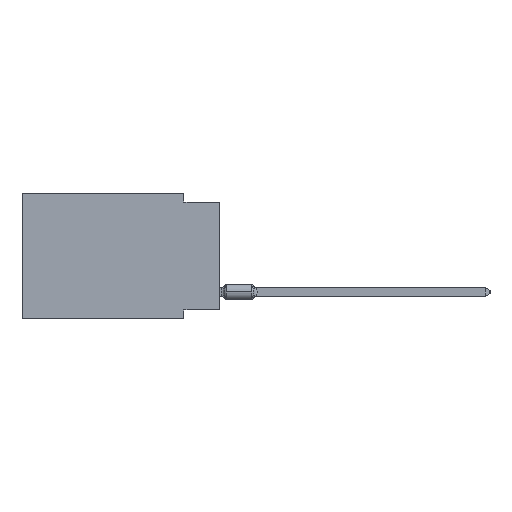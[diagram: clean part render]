
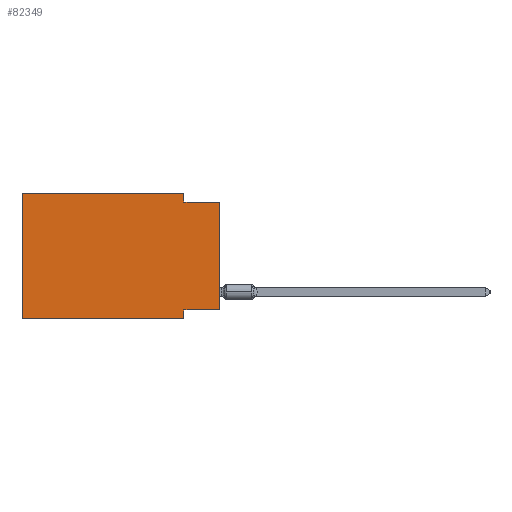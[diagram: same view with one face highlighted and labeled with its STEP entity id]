
A CAD part, left-side view. The second image highlights one B-rep face of the part: STEP entity #82349.
In plain terms, the highlighted planar face has unit normal (-1, 0, 0).
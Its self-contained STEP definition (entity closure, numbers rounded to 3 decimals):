
#4159 = VERTEX_POINT ( 'NONE', #14506 ) ;
#9010 = ORIENTED_EDGE ( 'NONE', *, *, #50529, .F. ) ;
#12058 = PLANE ( 'NONE',  #47801 ) ;
#12975 = DIRECTION ( 'NONE',  ( 0., 1., 0. ) ) ;
#14506 = CARTESIAN_POINT ( 'NONE',  ( 0., 0., -8.255 ) ) ;
#16788 = CARTESIAN_POINT ( 'NONE',  ( 0., 13.97, 0. ) ) ;
#21115 = FACE_OUTER_BOUND ( 'NONE', #97179, .T. ) ;
#21198 = VERTEX_POINT ( 'NONE', #81687 ) ;
#22297 = VECTOR ( 'NONE', #28663, 1000. ) ;
#22477 = LINE ( 'NONE', #42906, #79350 ) ;
#22899 = DIRECTION ( 'NONE',  ( 0., 0., -1. ) ) ;
#23203 = CARTESIAN_POINT ( 'NONE',  ( 0., 2.54, 0. ) ) ;
#23236 = ORIENTED_EDGE ( 'NONE', *, *, #86019, .T. ) ;
#24250 = DIRECTION ( 'NONE',  ( 0., 0., 1. ) ) ;
#24528 = CARTESIAN_POINT ( 'NONE',  ( 0., 2.54, -0.635 ) ) ;
#25127 = DIRECTION ( 'NONE',  ( 0., 0., -1. ) ) ;
#27028 = DIRECTION ( 'NONE',  ( 0., 0., 1. ) ) ;
#28663 = DIRECTION ( 'NONE',  ( 0., 0., -1. ) ) ;
#30539 = EDGE_CURVE ( 'NONE', #38605, #75224, #61893, .T. ) ;
#32677 = EDGE_CURVE ( 'NONE', #4159, #89477, #22477, .T. ) ;
#34767 = CARTESIAN_POINT ( 'NONE',  ( 0., 2.54, 0. ) ) ;
#36271 = CARTESIAN_POINT ( 'NONE',  ( 0., 0., -0.635 ) ) ;
#38147 = CARTESIAN_POINT ( 'NONE',  ( 0., 13.97, -8.89 ) ) ;
#38381 = EDGE_CURVE ( 'NONE', #4159, #113474, #112530, .T. ) ;
#38605 = VERTEX_POINT ( 'NONE', #23203 ) ;
#39523 = VECTOR ( 'NONE', #113791, 1000. ) ;
#39786 = CARTESIAN_POINT ( 'NONE',  ( 0., 13.97, 0. ) ) ;
#39924 = LINE ( 'NONE', #38147, #50037 ) ;
#41867 = VECTOR ( 'NONE', #25127, 1000. ) ;
#42906 = CARTESIAN_POINT ( 'NONE',  ( 0., 0., 0. ) ) ;
#47801 = AXIS2_PLACEMENT_3D ( 'NONE', #39786, #58480, #22899 ) ;
#48976 = DIRECTION ( 'NONE',  ( 0., -1., 0. ) ) ;
#50037 = VECTOR ( 'NONE', #48976, 1000. ) ;
#50529 = EDGE_CURVE ( 'NONE', #77059, #94277, #99419, .T. ) ;
#58480 = DIRECTION ( 'NONE',  ( 1., 0., 0. ) ) ;
#59437 = CARTESIAN_POINT ( 'NONE',  ( 0., 2.54, -8.255 ) ) ;
#61893 = LINE ( 'NONE', #34767, #41867 ) ;
#61899 = LINE ( 'NONE', #80033, #94812 ) ;
#62919 = CARTESIAN_POINT ( 'NONE',  ( 0., 13.97, -8.89 ) ) ;
#64763 = EDGE_CURVE ( 'NONE', #113474, #21198, #111313, .T. ) ;
#70947 = DIRECTION ( 'NONE',  ( 0., -1., 0. ) ) ;
#74313 = ORIENTED_EDGE ( 'NONE', *, *, #38381, .F. ) ;
#75224 = VERTEX_POINT ( 'NONE', #24528 ) ;
#76409 = LINE ( 'NONE', #113210, #39523 ) ;
#77059 = VERTEX_POINT ( 'NONE', #62919 ) ;
#77460 = VECTOR ( 'NONE', #27028, 1000. ) ;
#79196 = ORIENTED_EDGE ( 'NONE', *, *, #64763, .F. ) ;
#79350 = VECTOR ( 'NONE', #24250, 1000. ) ;
#80033 = CARTESIAN_POINT ( 'NONE',  ( 0., 13.97, 0. ) ) ;
#81687 = CARTESIAN_POINT ( 'NONE',  ( 0., 2.54, -8.89 ) ) ;
#81879 = ORIENTED_EDGE ( 'NONE', *, *, #103166, .F. ) ;
#82259 = ORIENTED_EDGE ( 'NONE', *, *, #32677, .T. ) ;
#82349 = ADVANCED_FACE ( 'NONE', ( #21115 ), #12058, .F. ) ;
#83552 = ORIENTED_EDGE ( 'NONE', *, *, #88549, .F. ) ;
#86019 = EDGE_CURVE ( 'NONE', #77059, #21198, #39924, .T. ) ;
#88549 = EDGE_CURVE ( 'NONE', #94277, #38605, #61899, .T. ) ;
#89477 = VERTEX_POINT ( 'NONE', #36271 ) ;
#91002 = ORIENTED_EDGE ( 'NONE', *, *, #30539, .F. ) ;
#94277 = VERTEX_POINT ( 'NONE', #119308 ) ;
#94812 = VECTOR ( 'NONE', #70947, 1000. ) ;
#97179 = EDGE_LOOP ( 'NONE', ( #82259, #81879, #91002, #83552, #9010, #23236, #79196, #74313 ) ) ;
#97344 = VECTOR ( 'NONE', #12975, 1000. ) ;
#99419 = LINE ( 'NONE', #16788, #77460 ) ;
#102878 = CARTESIAN_POINT ( 'NONE',  ( 0., 0., -8.255 ) ) ;
#103166 = EDGE_CURVE ( 'NONE', #75224, #89477, #76409, .T. ) ;
#111313 = LINE ( 'NONE', #118557, #22297 ) ;
#112530 = LINE ( 'NONE', #102878, #97344 ) ;
#113210 = CARTESIAN_POINT ( 'NONE',  ( 0., 0., -0.635 ) ) ;
#113474 = VERTEX_POINT ( 'NONE', #59437 ) ;
#113791 = DIRECTION ( 'NONE',  ( 0., -1., 0. ) ) ;
#118557 = CARTESIAN_POINT ( 'NONE',  ( 0., 2.54, -8.89 ) ) ;
#119308 = CARTESIAN_POINT ( 'NONE',  ( 0., 13.97, 0. ) ) ;
